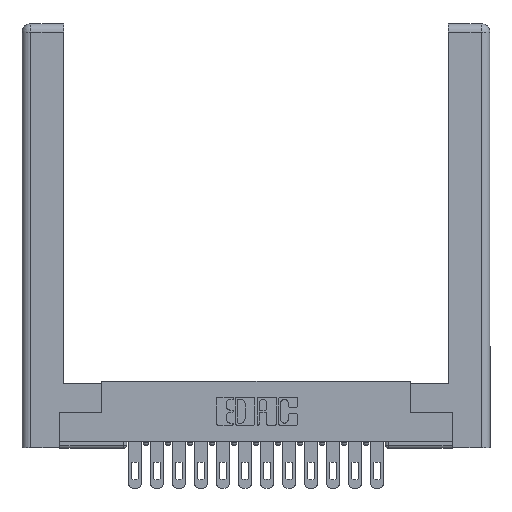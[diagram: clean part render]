
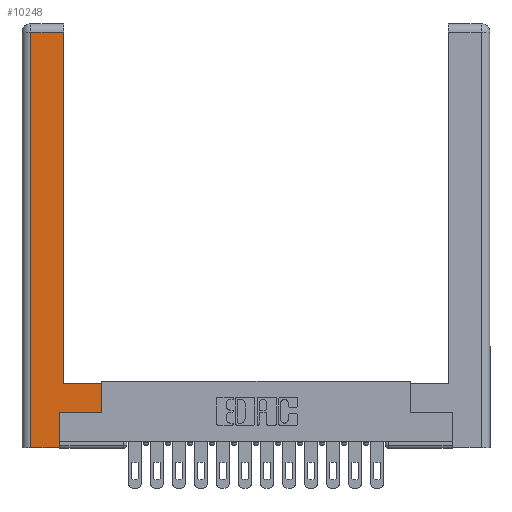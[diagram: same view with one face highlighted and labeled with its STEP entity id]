
A CAD part, top view. The second image highlights one B-rep face of the part: STEP entity #10248.
In plain terms, the highlighted planar face has unit normal (0, 0, 1).
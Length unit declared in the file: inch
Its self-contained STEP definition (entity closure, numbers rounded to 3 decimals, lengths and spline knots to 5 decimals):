
#348 = VECTOR ( 'NONE', #5391, 39.37008 ) ;
#473 = CARTESIAN_POINT ( 'NONE',  ( 0.565, 0.245, 0. ) ) ;
#512 = ORIENTED_EDGE ( 'NONE', *, *, #15615, .T. ) ;
#520 = FACE_OUTER_BOUND ( 'NONE', #1524, .T. ) ;
#730 = ORIENTED_EDGE ( 'NONE', *, *, #8885, .T. ) ;
#1056 = CARTESIAN_POINT ( 'NONE',  ( 0.0615, 2.94, 0. ) ) ;
#1516 = LINE ( 'NONE', #6171, #8155 ) ;
#1524 = EDGE_LOOP ( 'NONE', ( #730, #14605, #9519, #10931, #8166, #512, #3914, #6992 ) ) ;
#1712 = CARTESIAN_POINT ( 'NONE',  ( 0.565, 0.245, 0. ) ) ;
#2267 = DIRECTION ( 'NONE',  ( 0., -1., 0. ) ) ;
#2427 = CARTESIAN_POINT ( 'NONE',  ( 0.265, 0., 0. ) ) ;
#2520 = VERTEX_POINT ( 'NONE', #3050 ) ;
#2860 = VERTEX_POINT ( 'NONE', #1056 ) ;
#2891 = DIRECTION ( 'NONE',  ( 0., 0., -1. ) ) ;
#3050 = CARTESIAN_POINT ( 'NONE',  ( 0.0615, 0., 0. ) ) ;
#3272 = VERTEX_POINT ( 'NONE', #1712 ) ;
#3914 = ORIENTED_EDGE ( 'NONE', *, *, #3997, .T. ) ;
#3997 = EDGE_CURVE ( 'NONE', #3272, #11790, #10782, .T. ) ;
#4670 = VERTEX_POINT ( 'NONE', #11647 ) ;
#4896 = DIRECTION ( 'NONE',  ( -1., 0., 0. ) ) ;
#5343 = VECTOR ( 'NONE', #14062, 39.37008 ) ;
#5391 = DIRECTION ( 'NONE',  ( 0., 1., 0. ) ) ;
#5570 = DIRECTION ( 'NONE',  ( 1., 0., 0. ) ) ;
#5831 = LINE ( 'NONE', #10034, #16056 ) ;
#6171 = CARTESIAN_POINT ( 'NONE',  ( 0.0615, 2.94, 0. ) ) ;
#6468 = CARTESIAN_POINT ( 'NONE',  ( 0.295, 3., 0. ) ) ;
#6479 = EDGE_CURVE ( 'NONE', #11790, #8725, #5831, .T. ) ;
#6858 = EDGE_CURVE ( 'NONE', #2520, #8737, #13033, .T. ) ;
#6992 = ORIENTED_EDGE ( 'NONE', *, *, #6479, .T. ) ;
#7194 = LINE ( 'NONE', #6468, #348 ) ;
#7409 = CARTESIAN_POINT ( 'NONE',  ( 0.265, 0., 0. ) ) ;
#7467 = LINE ( 'NONE', #11380, #12422 ) ;
#7478 = VECTOR ( 'NONE', #5570, 39.37008 ) ;
#7503 = DIRECTION ( 'NONE',  ( -1., 0., 0. ) ) ;
#7612 = VECTOR ( 'NONE', #16586, 39.37008 ) ;
#8155 = VECTOR ( 'NONE', #7503, 39.37008 ) ;
#8166 = ORIENTED_EDGE ( 'NONE', *, *, #8670, .T. ) ;
#8670 = EDGE_CURVE ( 'NONE', #8737, #4670, #9374, .T. ) ;
#8725 = VERTEX_POINT ( 'NONE', #11434 ) ;
#8737 = VERTEX_POINT ( 'NONE', #2427 ) ;
#8885 = EDGE_CURVE ( 'NONE', #8725, #13695, #7194, .T. ) ;
#9374 = LINE ( 'NONE', #12530, #5343 ) ;
#9519 = ORIENTED_EDGE ( 'NONE', *, *, #12610, .T. ) ;
#9778 = AXIS2_PLACEMENT_3D ( 'NONE', #13091, #2891, #11993 ) ;
#10034 = CARTESIAN_POINT ( 'NONE',  ( 0.295, 0.45, 0. ) ) ;
#10248 = ADVANCED_FACE ( 'NONE', ( #520 ), #11831, .F. ) ;
#10564 = CARTESIAN_POINT ( 'NONE',  ( 0.565, 0.45, 0. ) ) ;
#10782 = LINE ( 'NONE', #10564, #14383 ) ;
#10931 = ORIENTED_EDGE ( 'NONE', *, *, #6858, .T. ) ;
#11380 = CARTESIAN_POINT ( 'NONE',  ( 0.0615, 0., 0. ) ) ;
#11434 = CARTESIAN_POINT ( 'NONE',  ( 0.295, 0.45, 0. ) ) ;
#11647 = CARTESIAN_POINT ( 'NONE',  ( 0.265, 0.245, 0. ) ) ;
#11790 = VERTEX_POINT ( 'NONE', #15734 ) ;
#11831 = PLANE ( 'NONE',  #9778 ) ;
#11993 = DIRECTION ( 'NONE',  ( -1., 0., 0. ) ) ;
#12422 = VECTOR ( 'NONE', #2267, 39.37008 ) ;
#12530 = CARTESIAN_POINT ( 'NONE',  ( 0.265, 0.245, 0. ) ) ;
#12610 = EDGE_CURVE ( 'NONE', #2860, #2520, #7467, .T. ) ;
#13033 = LINE ( 'NONE', #7409, #7612 ) ;
#13091 = CARTESIAN_POINT ( 'NONE',  ( 0., 0., 0. ) ) ;
#13695 = VERTEX_POINT ( 'NONE', #13751 ) ;
#13751 = CARTESIAN_POINT ( 'NONE',  ( 0.295, 2.94, 0. ) ) ;
#13872 = EDGE_CURVE ( 'NONE', #13695, #2860, #1516, .T. ) ;
#13924 = LINE ( 'NONE', #473, #7478 ) ;
#14062 = DIRECTION ( 'NONE',  ( 0., 1., 0. ) ) ;
#14383 = VECTOR ( 'NONE', #14473, 39.37008 ) ;
#14473 = DIRECTION ( 'NONE',  ( 0., 1., 0. ) ) ;
#14605 = ORIENTED_EDGE ( 'NONE', *, *, #13872, .T. ) ;
#15615 = EDGE_CURVE ( 'NONE', #4670, #3272, #13924, .T. ) ;
#15734 = CARTESIAN_POINT ( 'NONE',  ( 0.565, 0.45, 0. ) ) ;
#16056 = VECTOR ( 'NONE', #4896, 39.37008 ) ;
#16586 = DIRECTION ( 'NONE',  ( 1., 0., 0. ) ) ;
